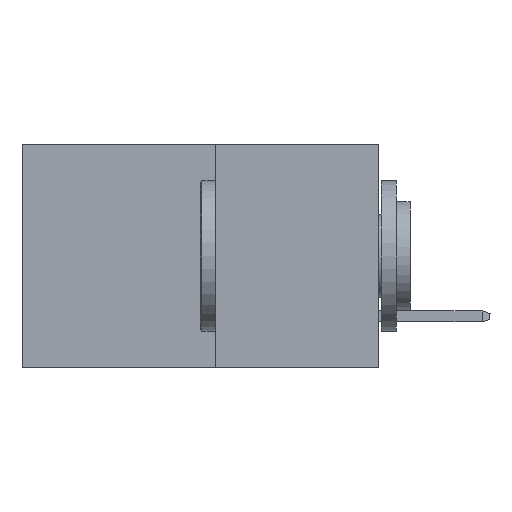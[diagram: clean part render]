
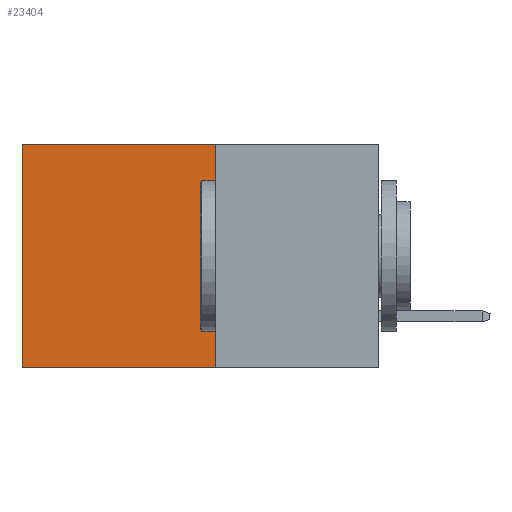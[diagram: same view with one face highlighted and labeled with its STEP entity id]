
A CAD part, left-side view. The second image highlights one B-rep face of the part: STEP entity #23404.
In plain terms, the highlighted planar face has unit normal (-1, 0, 0).
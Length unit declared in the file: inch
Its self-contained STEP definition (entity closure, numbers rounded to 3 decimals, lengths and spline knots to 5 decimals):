
#777 = VECTOR ( 'NONE', #6588, 39.37008 ) ;
#1054 = CARTESIAN_POINT ( 'NONE',  ( 0.277, 0.27, -0.37 ) ) ;
#3024 = CARTESIAN_POINT ( 'NONE',  ( 0.277, 0.59, -0.37 ) ) ;
#3331 = VECTOR ( 'NONE', #23252, 39.37008 ) ;
#4181 = LINE ( 'NONE', #1054, #23775 ) ;
#5747 = CARTESIAN_POINT ( 'NONE',  ( 0.277, 0.27, -0.37 ) ) ;
#6138 = LINE ( 'NONE', #3024, #21192 ) ;
#6148 = LINE ( 'NONE', #17873, #777 ) ;
#6320 = ORIENTED_EDGE ( 'NONE', *, *, #7820, .F. ) ;
#6588 = DIRECTION ( 'NONE',  ( 0., 0., -1. ) ) ;
#6705 = CARTESIAN_POINT ( 'NONE',  ( 0.277, 0.27, 0. ) ) ;
#6971 = CARTESIAN_POINT ( 'NONE',  ( 0.277, 0.27, -0.37 ) ) ;
#7679 = DIRECTION ( 'NONE',  ( 0., 0., -1. ) ) ;
#7710 = EDGE_CURVE ( 'NONE', #14968, #22830, #13527, .T. ) ;
#7820 = EDGE_CURVE ( 'NONE', #14968, #14454, #6148, .T. ) ;
#8188 = CARTESIAN_POINT ( 'NONE',  ( 0.277, 0.27, 0. ) ) ;
#8420 = FACE_OUTER_BOUND ( 'NONE', #12507, .T. ) ;
#9314 = ORIENTED_EDGE ( 'NONE', *, *, #18886, .T. ) ;
#10688 = ORIENTED_EDGE ( 'NONE', *, *, #7710, .T. ) ;
#10762 = AXIS2_PLACEMENT_3D ( 'NONE', #5747, #18973, #7679 ) ;
#11407 = PLANE ( 'NONE',  #10762 ) ;
#12507 = EDGE_LOOP ( 'NONE', ( #9314, #21233, #6320, #10688 ) ) ;
#13527 = LINE ( 'NONE', #8188, #3331 ) ;
#13582 = CARTESIAN_POINT ( 'NONE',  ( 0.277, 0.59, -0.37 ) ) ;
#14454 = VERTEX_POINT ( 'NONE', #6971 ) ;
#14968 = VERTEX_POINT ( 'NONE', #6705 ) ;
#17873 = CARTESIAN_POINT ( 'NONE',  ( 0.277, 0.27, -0.37 ) ) ;
#18238 = DIRECTION ( 'NONE',  ( 0., 0., -1. ) ) ;
#18886 = EDGE_CURVE ( 'NONE', #22830, #23526, #6138, .T. ) ;
#18973 = DIRECTION ( 'NONE',  ( 1., 0., 0. ) ) ;
#20277 = DIRECTION ( 'NONE',  ( 0., 1., 0. ) ) ;
#20937 = EDGE_CURVE ( 'NONE', #14454, #23526, #4181, .T. ) ;
#21192 = VECTOR ( 'NONE', #18238, 39.37008 ) ;
#21233 = ORIENTED_EDGE ( 'NONE', *, *, #20937, .F. ) ;
#22830 = VERTEX_POINT ( 'NONE', #22904 ) ;
#22904 = CARTESIAN_POINT ( 'NONE',  ( 0.277, 0.59, 0. ) ) ;
#23252 = DIRECTION ( 'NONE',  ( 0., 1., 0. ) ) ;
#23404 = ADVANCED_FACE ( 'NONE', ( #8420 ), #11407, .F. ) ;
#23526 = VERTEX_POINT ( 'NONE', #13582 ) ;
#23775 = VECTOR ( 'NONE', #20277, 39.37008 ) ;
